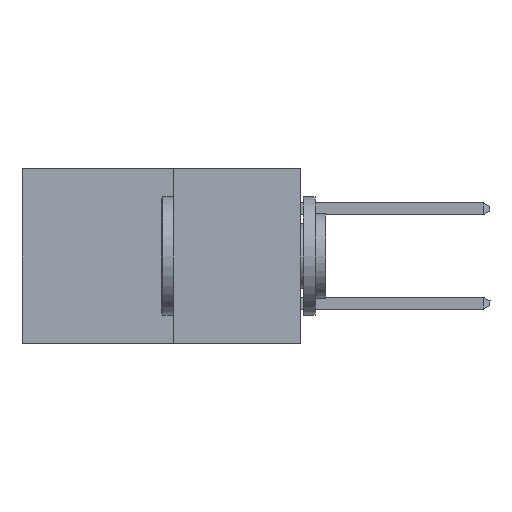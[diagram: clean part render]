
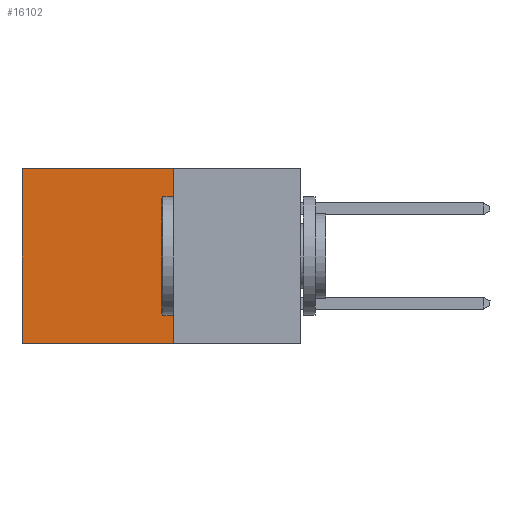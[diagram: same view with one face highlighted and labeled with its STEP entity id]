
A CAD part, left-side view. The second image highlights one B-rep face of the part: STEP entity #16102.
In plain terms, the highlighted planar face has unit normal (-1, 0, 0).
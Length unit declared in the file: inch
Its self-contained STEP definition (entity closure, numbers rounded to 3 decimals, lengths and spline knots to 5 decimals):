
#140 = DIRECTION ( 'NONE',  ( 0., 0., -1. ) ) ;
#945 = EDGE_CURVE ( 'NONE', #5531, #20964, #17057, .T. ) ;
#1269 = VECTOR ( 'NONE', #140, 39.37008 ) ;
#2316 = LINE ( 'NONE', #8734, #1269 ) ;
#3252 = CARTESIAN_POINT ( 'NONE',  ( 0.277, 0.27, -0.37 ) ) ;
#3546 = ORIENTED_EDGE ( 'NONE', *, *, #8425, .F. ) ;
#3579 = VERTEX_POINT ( 'NONE', #13279 ) ;
#3738 = VECTOR ( 'NONE', #10921, 39.37008 ) ;
#3969 = ORIENTED_EDGE ( 'NONE', *, *, #16555, .T. ) ;
#5531 = VERTEX_POINT ( 'NONE', #8500 ) ;
#7933 = CARTESIAN_POINT ( 'NONE',  ( 0.277, 0.59, 0. ) ) ;
#8076 = CARTESIAN_POINT ( 'NONE',  ( 0.277, 0.27, -0.37 ) ) ;
#8140 = DIRECTION ( 'NONE',  ( 1., 0., 0. ) ) ;
#8425 = EDGE_CURVE ( 'NONE', #16205, #3579, #13382, .T. ) ;
#8500 = CARTESIAN_POINT ( 'NONE',  ( 0.277, 0.27, 0. ) ) ;
#8734 = CARTESIAN_POINT ( 'NONE',  ( 0.277, 0.27, -0.37 ) ) ;
#10604 = DIRECTION ( 'NONE',  ( 0., 1., 0. ) ) ;
#10776 = CARTESIAN_POINT ( 'NONE',  ( 0.277, 0.27, -0.37 ) ) ;
#10777 = VECTOR ( 'NONE', #10849, 39.37008 ) ;
#10849 = DIRECTION ( 'NONE',  ( 0., 0., -1. ) ) ;
#10921 = DIRECTION ( 'NONE',  ( 0., 1., 0. ) ) ;
#11551 = CARTESIAN_POINT ( 'NONE',  ( 0.277, 0.27, 0. ) ) ;
#11817 = EDGE_LOOP ( 'NONE', ( #3969, #3546, #16643, #14176 ) ) ;
#13279 = CARTESIAN_POINT ( 'NONE',  ( 0.277, 0.59, -0.37 ) ) ;
#13382 = LINE ( 'NONE', #10776, #13900 ) ;
#13900 = VECTOR ( 'NONE', #10604, 39.37008 ) ;
#14176 = ORIENTED_EDGE ( 'NONE', *, *, #945, .T. ) ;
#16102 = ADVANCED_FACE ( 'NONE', ( #19537 ), #16345, .F. ) ;
#16205 = VERTEX_POINT ( 'NONE', #3252 ) ;
#16345 = PLANE ( 'NONE',  #16553 ) ;
#16553 = AXIS2_PLACEMENT_3D ( 'NONE', #8076, #8140, #19538 ) ;
#16555 = EDGE_CURVE ( 'NONE', #20964, #3579, #19356, .T. ) ;
#16643 = ORIENTED_EDGE ( 'NONE', *, *, #20660, .F. ) ;
#17057 = LINE ( 'NONE', #11551, #3738 ) ;
#18976 = CARTESIAN_POINT ( 'NONE',  ( 0.277, 0.59, -0.37 ) ) ;
#19356 = LINE ( 'NONE', #18976, #10777 ) ;
#19537 = FACE_OUTER_BOUND ( 'NONE', #11817, .T. ) ;
#19538 = DIRECTION ( 'NONE',  ( 0., 0., -1. ) ) ;
#20660 = EDGE_CURVE ( 'NONE', #5531, #16205, #2316, .T. ) ;
#20964 = VERTEX_POINT ( 'NONE', #7933 ) ;
